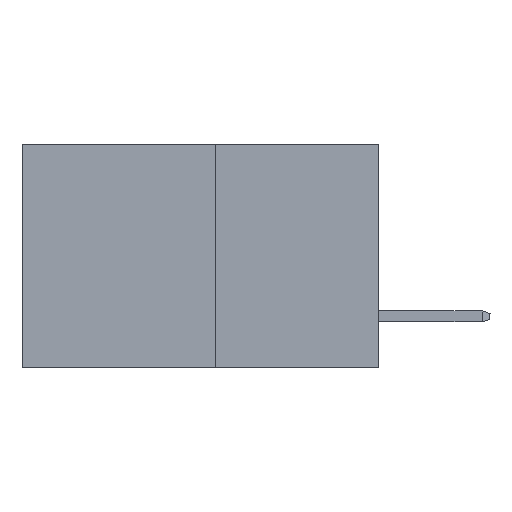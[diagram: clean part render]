
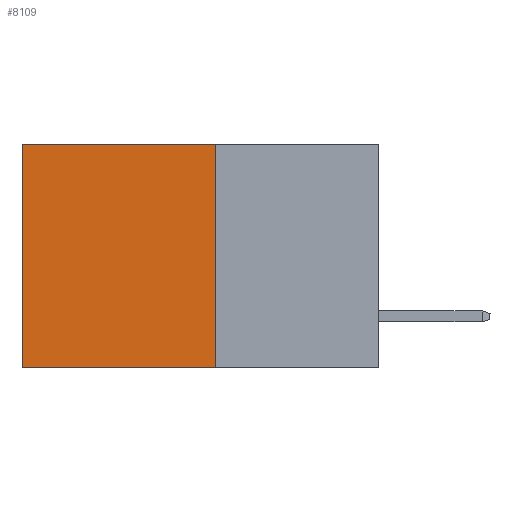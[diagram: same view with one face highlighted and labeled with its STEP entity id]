
A CAD part, left-side view. The second image highlights one B-rep face of the part: STEP entity #8109.
In plain terms, the highlighted planar face has unit normal (-1, 0, 0).
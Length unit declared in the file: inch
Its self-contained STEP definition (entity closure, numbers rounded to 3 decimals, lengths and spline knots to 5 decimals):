
#122 = CARTESIAN_POINT ( 'NONE',  ( 0.277, 0.27, 0. ) ) ;
#227 = DIRECTION ( 'NONE',  ( 0., 1., 0. ) ) ;
#1233 = DIRECTION ( 'NONE',  ( 0., 1., 0. ) ) ;
#1685 = AXIS2_PLACEMENT_3D ( 'NONE', #11361, #4846, #12458 ) ;
#2098 = FACE_OUTER_BOUND ( 'NONE', #3785, .T. ) ;
#2200 = CARTESIAN_POINT ( 'NONE',  ( 0.277, 0.59, 0. ) ) ;
#2621 = VERTEX_POINT ( 'NONE', #9671 ) ;
#2921 = VERTEX_POINT ( 'NONE', #6956 ) ;
#3175 = VECTOR ( 'NONE', #1233, 39.37008 ) ;
#3453 = CARTESIAN_POINT ( 'NONE',  ( 0.277, 0.27, -0.37 ) ) ;
#3740 = VECTOR ( 'NONE', #4261, 39.37008 ) ;
#3785 = EDGE_LOOP ( 'NONE', ( #4308, #12564, #12330, #12188 ) ) ;
#3881 = LINE ( 'NONE', #3453, #3175 ) ;
#4084 = VECTOR ( 'NONE', #227, 39.37008 ) ;
#4177 = DIRECTION ( 'NONE',  ( 0., 0., -1. ) ) ;
#4261 = DIRECTION ( 'NONE',  ( 0., 0., -1. ) ) ;
#4275 = CARTESIAN_POINT ( 'NONE',  ( 0.277, 0.59, -0.37 ) ) ;
#4308 = ORIENTED_EDGE ( 'NONE', *, *, #5168, .T. ) ;
#4846 = DIRECTION ( 'NONE',  ( 1., 0., 0. ) ) ;
#5168 = EDGE_CURVE ( 'NONE', #12800, #2621, #12780, .T. ) ;
#5549 = EDGE_CURVE ( 'NONE', #2921, #12800, #7693, .T. ) ;
#6956 = CARTESIAN_POINT ( 'NONE',  ( 0.277, 0.27, 0. ) ) ;
#7293 = VECTOR ( 'NONE', #4177, 39.37008 ) ;
#7693 = LINE ( 'NONE', #122, #4084 ) ;
#7727 = EDGE_CURVE ( 'NONE', #2921, #9837, #10512, .T. ) ;
#7897 = CARTESIAN_POINT ( 'NONE',  ( 0.277, 0.27, -0.37 ) ) ;
#8109 = ADVANCED_FACE ( 'NONE', ( #2098 ), #9189, .F. ) ;
#9189 = PLANE ( 'NONE',  #1685 ) ;
#9671 = CARTESIAN_POINT ( 'NONE',  ( 0.277, 0.59, -0.37 ) ) ;
#9837 = VERTEX_POINT ( 'NONE', #7897 ) ;
#10512 = LINE ( 'NONE', #11794, #7293 ) ;
#11361 = CARTESIAN_POINT ( 'NONE',  ( 0.277, 0.27, -0.37 ) ) ;
#11794 = CARTESIAN_POINT ( 'NONE',  ( 0.277, 0.27, -0.37 ) ) ;
#12188 = ORIENTED_EDGE ( 'NONE', *, *, #5549, .T. ) ;
#12330 = ORIENTED_EDGE ( 'NONE', *, *, #7727, .F. ) ;
#12458 = DIRECTION ( 'NONE',  ( 0., 0., -1. ) ) ;
#12564 = ORIENTED_EDGE ( 'NONE', *, *, #13546, .F. ) ;
#12780 = LINE ( 'NONE', #4275, #3740 ) ;
#12800 = VERTEX_POINT ( 'NONE', #2200 ) ;
#13546 = EDGE_CURVE ( 'NONE', #9837, #2621, #3881, .T. ) ;
